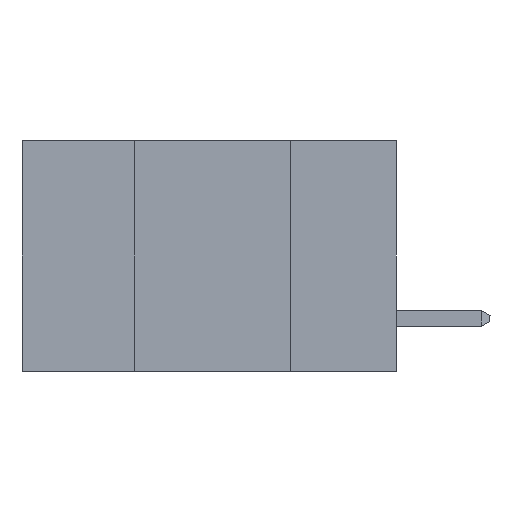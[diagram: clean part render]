
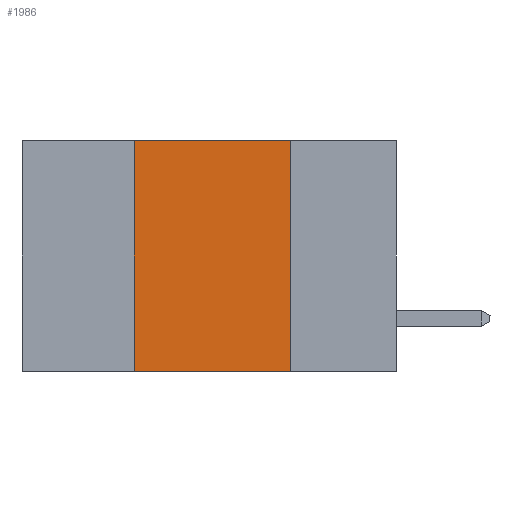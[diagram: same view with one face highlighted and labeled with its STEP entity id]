
A CAD part, left-side view. The second image highlights one B-rep face of the part: STEP entity #1986.
In plain terms, the highlighted planar face has unit normal (-1, 0, 0).
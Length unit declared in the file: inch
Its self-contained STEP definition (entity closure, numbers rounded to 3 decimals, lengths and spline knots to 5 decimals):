
#1986 = ADVANCED_FACE ( 'NONE', ( #5685 ), #3515, .F. ) ;
#3076 = EDGE_CURVE ( 'NONE', #18374, #4890, #5312, .T. ) ;
#3464 = DIRECTION ( 'NONE',  ( 0., 0., -1. ) ) ;
#3490 = DIRECTION ( 'NONE',  ( 1., 0., 0. ) ) ;
#3515 = PLANE ( 'NONE',  #24662 ) ;
#3821 = CARTESIAN_POINT ( 'NONE',  ( 0., 0.6, 0. ) ) ;
#3879 = EDGE_LOOP ( 'NONE', ( #16912, #4115, #23448, #8168 ) ) ;
#3892 = LINE ( 'NONE', #16973, #24770 ) ;
#4115 = ORIENTED_EDGE ( 'NONE', *, *, #14622, .F. ) ;
#4723 = LINE ( 'NONE', #9504, #8887 ) ;
#4890 = VERTEX_POINT ( 'NONE', #6775 ) ;
#5312 = LINE ( 'NONE', #6058, #16809 ) ;
#5685 = FACE_OUTER_BOUND ( 'NONE', #3879, .T. ) ;
#6058 = CARTESIAN_POINT ( 'NONE',  ( 0., 0.42, -0.37 ) ) ;
#6090 = DIRECTION ( 'NONE',  ( 0., 0., 1. ) ) ;
#6521 = CARTESIAN_POINT ( 'NONE',  ( 0., 0.17, 0. ) ) ;
#6775 = CARTESIAN_POINT ( 'NONE',  ( 0., 0.42, 0. ) ) ;
#7556 = CARTESIAN_POINT ( 'NONE',  ( 0., 0.42, -0.37 ) ) ;
#8168 = ORIENTED_EDGE ( 'NONE', *, *, #18109, .T. ) ;
#8887 = VECTOR ( 'NONE', #21587, 39.37008 ) ;
#9504 = CARTESIAN_POINT ( 'NONE',  ( 0., 0.6, 0. ) ) ;
#10501 = CARTESIAN_POINT ( 'NONE',  ( 0., 0.17, -0.37 ) ) ;
#12475 = LINE ( 'NONE', #10501, #22504 ) ;
#14274 = EDGE_CURVE ( 'NONE', #18041, #15570, #12475, .T. ) ;
#14622 = EDGE_CURVE ( 'NONE', #4890, #18041, #4723, .T. ) ;
#15570 = VERTEX_POINT ( 'NONE', #18807 ) ;
#16809 = VECTOR ( 'NONE', #6090, 39.37008 ) ;
#16912 = ORIENTED_EDGE ( 'NONE', *, *, #14274, .F. ) ;
#16973 = CARTESIAN_POINT ( 'NONE',  ( 0., 0.6, -0.37 ) ) ;
#18041 = VERTEX_POINT ( 'NONE', #6521 ) ;
#18109 = EDGE_CURVE ( 'NONE', #18374, #15570, #3892, .T. ) ;
#18374 = VERTEX_POINT ( 'NONE', #7556 ) ;
#18807 = CARTESIAN_POINT ( 'NONE',  ( 0., 0.17, -0.37 ) ) ;
#20884 = DIRECTION ( 'NONE',  ( 0., -1., 0. ) ) ;
#21587 = DIRECTION ( 'NONE',  ( 0., -1., 0. ) ) ;
#22504 = VECTOR ( 'NONE', #24528, 39.37008 ) ;
#23448 = ORIENTED_EDGE ( 'NONE', *, *, #3076, .F. ) ;
#24528 = DIRECTION ( 'NONE',  ( 0., 0., -1. ) ) ;
#24662 = AXIS2_PLACEMENT_3D ( 'NONE', #3821, #3490, #3464 ) ;
#24770 = VECTOR ( 'NONE', #20884, 39.37008 ) ;
